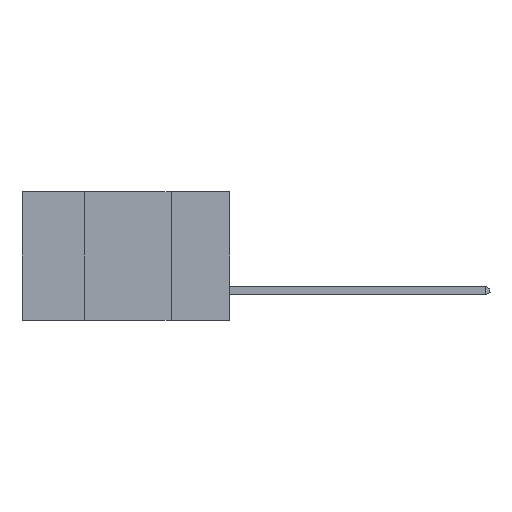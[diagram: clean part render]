
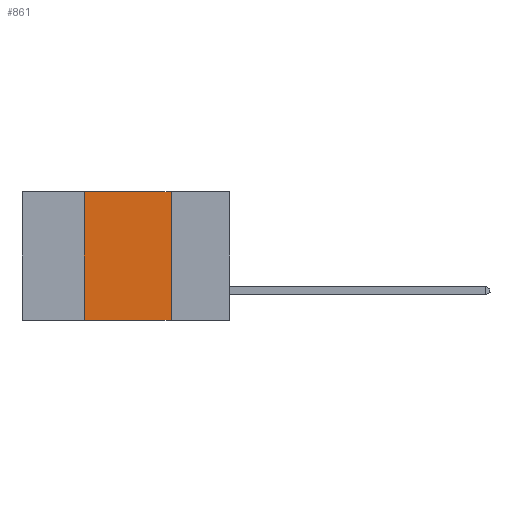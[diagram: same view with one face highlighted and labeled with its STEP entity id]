
A CAD part, left-side view. The second image highlights one B-rep face of the part: STEP entity #861.
In plain terms, the highlighted planar face has unit normal (-1, 0, 0).
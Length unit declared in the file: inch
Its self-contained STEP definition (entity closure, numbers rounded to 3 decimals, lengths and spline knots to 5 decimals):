
#227 = CARTESIAN_POINT ( 'NONE',  ( 0., 0.42, 0. ) ) ;
#353 = CARTESIAN_POINT ( 'NONE',  ( 0., 0.42, -0.37 ) ) ;
#674 = ORIENTED_EDGE ( 'NONE', *, *, #2714, .F. ) ;
#704 = VERTEX_POINT ( 'NONE', #7221 ) ;
#861 = ADVANCED_FACE ( 'NONE', ( #4666 ), #8329, .F. ) ;
#870 = VECTOR ( 'NONE', #1194, 39.37008 ) ;
#1194 = DIRECTION ( 'NONE',  ( 0., 0., 1. ) ) ;
#1347 = VECTOR ( 'NONE', #7651, 39.37008 ) ;
#1563 = CARTESIAN_POINT ( 'NONE',  ( 0., 0.6, -0.37 ) ) ;
#2203 = EDGE_CURVE ( 'NONE', #3927, #704, #7800, .T. ) ;
#2215 = LINE ( 'NONE', #1563, #3106 ) ;
#2383 = EDGE_CURVE ( 'NONE', #3870, #3927, #9569, .T. ) ;
#2428 = DIRECTION ( 'NONE',  ( 0., -1., 0. ) ) ;
#2613 = DIRECTION ( 'NONE',  ( 0., 0., -1. ) ) ;
#2714 = EDGE_CURVE ( 'NONE', #704, #6071, #8682, .T. ) ;
#3106 = VECTOR ( 'NONE', #7278, 39.37008 ) ;
#3370 = DIRECTION ( 'NONE',  ( 1., 0., 0. ) ) ;
#3870 = VERTEX_POINT ( 'NONE', #353 ) ;
#3927 = VERTEX_POINT ( 'NONE', #6026 ) ;
#4666 = FACE_OUTER_BOUND ( 'NONE', #8109, .T. ) ;
#6026 = CARTESIAN_POINT ( 'NONE',  ( 0., 0.42, 0. ) ) ;
#6071 = VERTEX_POINT ( 'NONE', #9576 ) ;
#6555 = ORIENTED_EDGE ( 'NONE', *, *, #2383, .F. ) ;
#7221 = CARTESIAN_POINT ( 'NONE',  ( 0., 0.17, 0. ) ) ;
#7278 = DIRECTION ( 'NONE',  ( 0., -1., 0. ) ) ;
#7651 = DIRECTION ( 'NONE',  ( 0., 0., -1. ) ) ;
#7800 = LINE ( 'NONE', #8142, #8821 ) ;
#7870 = ORIENTED_EDGE ( 'NONE', *, *, #10052, .T. ) ;
#8109 = EDGE_LOOP ( 'NONE', ( #674, #8167, #6555, #7870 ) ) ;
#8142 = CARTESIAN_POINT ( 'NONE',  ( 0., 0.6, 0. ) ) ;
#8167 = ORIENTED_EDGE ( 'NONE', *, *, #2203, .F. ) ;
#8329 = PLANE ( 'NONE',  #8948 ) ;
#8682 = LINE ( 'NONE', #10135, #1347 ) ;
#8821 = VECTOR ( 'NONE', #2428, 39.37008 ) ;
#8948 = AXIS2_PLACEMENT_3D ( 'NONE', #9873, #3370, #2613 ) ;
#9569 = LINE ( 'NONE', #227, #870 ) ;
#9576 = CARTESIAN_POINT ( 'NONE',  ( 0., 0.17, -0.37 ) ) ;
#9873 = CARTESIAN_POINT ( 'NONE',  ( 0., 0.6, 0. ) ) ;
#10052 = EDGE_CURVE ( 'NONE', #3870, #6071, #2215, .T. ) ;
#10135 = CARTESIAN_POINT ( 'NONE',  ( 0., 0.17, 0. ) ) ;
